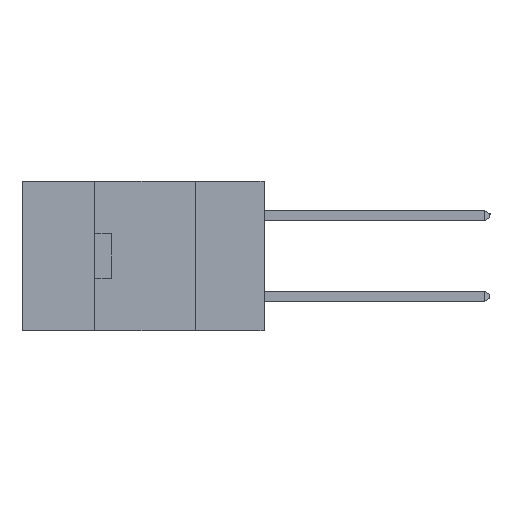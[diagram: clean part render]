
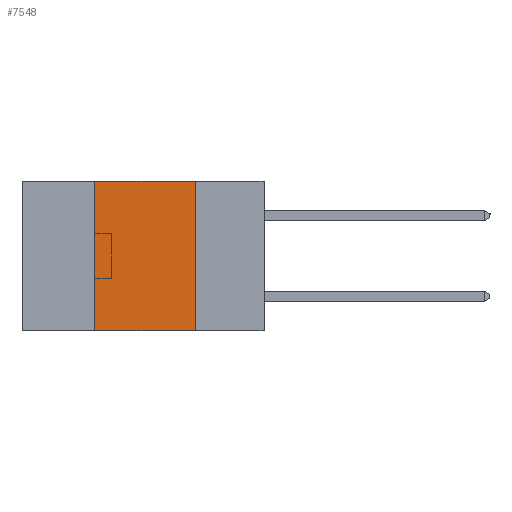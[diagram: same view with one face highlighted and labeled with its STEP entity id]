
A CAD part, left-side view. The second image highlights one B-rep face of the part: STEP entity #7548.
In plain terms, the highlighted planar face has unit normal (-1, 0, 0).
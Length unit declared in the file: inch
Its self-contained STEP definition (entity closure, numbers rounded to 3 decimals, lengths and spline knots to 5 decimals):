
#53 = VECTOR ( 'NONE', #18994, 39.37008 ) ;
#588 = LINE ( 'NONE', #15994, #10118 ) ;
#2446 = CARTESIAN_POINT ( 'NONE',  ( 0., 0.17, -0.37 ) ) ;
#2945 = VERTEX_POINT ( 'NONE', #19442 ) ;
#3219 = LINE ( 'NONE', #18327, #53 ) ;
#4184 = DIRECTION ( 'NONE',  ( 0., -1., 0. ) ) ;
#5487 = EDGE_CURVE ( 'NONE', #2945, #24919, #23481, .T. ) ;
#5825 = PLANE ( 'NONE',  #18923 ) ;
#7237 = CARTESIAN_POINT ( 'NONE',  ( 0., 0.42, 0. ) ) ;
#7465 = ORIENTED_EDGE ( 'NONE', *, *, #18367, .F. ) ;
#7477 = DIRECTION ( 'NONE',  ( 0., 0., 1. ) ) ;
#7548 = ADVANCED_FACE ( 'NONE', ( #7953 ), #5825, .F. ) ;
#7596 = ORIENTED_EDGE ( 'NONE', *, *, #9988, .F. ) ;
#7953 = FACE_OUTER_BOUND ( 'NONE', #16828, .T. ) ;
#8093 = DIRECTION ( 'NONE',  ( 0., 0., -1. ) ) ;
#9225 = DIRECTION ( 'NONE',  ( 0., -1., 0. ) ) ;
#9355 = ORIENTED_EDGE ( 'NONE', *, *, #27070, .F. ) ;
#9988 = EDGE_CURVE ( 'NONE', #14482, #22943, #588, .T. ) ;
#10118 = VECTOR ( 'NONE', #9225, 39.37008 ) ;
#14398 = CARTESIAN_POINT ( 'NONE',  ( 0., 0.42, -0.37 ) ) ;
#14482 = VERTEX_POINT ( 'NONE', #7237 ) ;
#15765 = VECTOR ( 'NONE', #7477, 39.37008 ) ;
#15994 = CARTESIAN_POINT ( 'NONE',  ( 0., 0.6, 0. ) ) ;
#16828 = EDGE_LOOP ( 'NONE', ( #9355, #7596, #7465, #18727 ) ) ;
#18327 = CARTESIAN_POINT ( 'NONE',  ( 0., 0.17, -0.37 ) ) ;
#18367 = EDGE_CURVE ( 'NONE', #2945, #14482, #27220, .T. ) ;
#18727 = ORIENTED_EDGE ( 'NONE', *, *, #5487, .T. ) ;
#18923 = AXIS2_PLACEMENT_3D ( 'NONE', #23006, #27412, #8093 ) ;
#18994 = DIRECTION ( 'NONE',  ( 0., 0., -1. ) ) ;
#19442 = CARTESIAN_POINT ( 'NONE',  ( 0., 0.42, -0.37 ) ) ;
#20541 = CARTESIAN_POINT ( 'NONE',  ( 0., 0.17, 0. ) ) ;
#22943 = VERTEX_POINT ( 'NONE', #20541 ) ;
#23006 = CARTESIAN_POINT ( 'NONE',  ( 0., 0.6, 0. ) ) ;
#23481 = LINE ( 'NONE', #25904, #26034 ) ;
#24919 = VERTEX_POINT ( 'NONE', #2446 ) ;
#25904 = CARTESIAN_POINT ( 'NONE',  ( 0., 0.6, -0.37 ) ) ;
#26034 = VECTOR ( 'NONE', #4184, 39.37008 ) ;
#27070 = EDGE_CURVE ( 'NONE', #22943, #24919, #3219, .T. ) ;
#27220 = LINE ( 'NONE', #14398, #15765 ) ;
#27412 = DIRECTION ( 'NONE',  ( 1., 0., 0. ) ) ;
